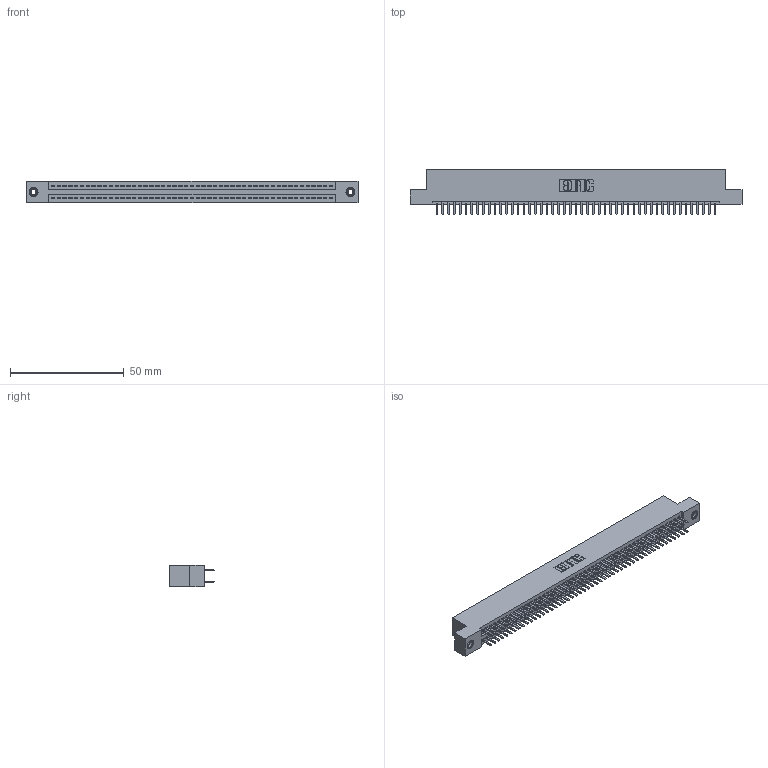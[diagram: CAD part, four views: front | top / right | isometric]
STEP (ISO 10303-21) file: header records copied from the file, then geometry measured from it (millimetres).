
FILE_DESCRIPTION (( 'STEP AP203' ), '1' );
FILE_NAME ('395-098-520-208.STEP', '2018-11-29T18:37:06', ( '' ), ( '' ), 'SwSTEP 2.0', 'SolidWorks 2016', '' );
FILE_SCHEMA (( 'CONFIG_CONTROL_DESIGN' ));
Length unit declared in the file: inch
Products named in the file (4): 395-098-520-208; 345-250-001_345-250-003-102; 345-292-001_345-293-120; 345 Part_Flush Mounting Lugs - 0.156 Dia-TI
Assembly tree (101 placements, depth 2):
  395-098-520-208
    345 Part_Flush Mounting Lugs - 0.156 Dia-TI
    345-292-001_345-293-120  x98
    345-250-001_345-250-003-102  x2
Bounding box: 145.67 x 19.68 x 9.4 mm (x, y, z)
Volume: 14165.8 mm3; surface area: 20996.8 mm2
Topology: 101 solids, 101 shells, 5478 faces, 15863 edges, 10306 vertices
Faces by surface type: plane 3542, cylinder 1920, cone 12, torus 4
Entity records: 38804 total; most frequent: CARTESIAN_POINT 6491, ORIENTED_EDGE 6406, DIRECTION 5729, EDGE_CURVE 3203, VECTOR 2851, LINE 2851, VERTEX_POINT 2128, AXIS2_PLACEMENT_3D 1439
